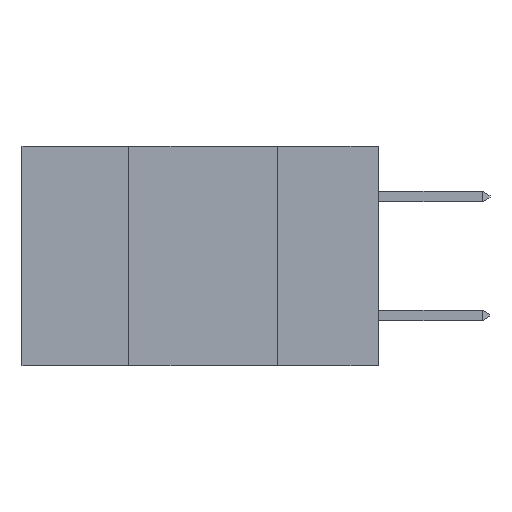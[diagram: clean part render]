
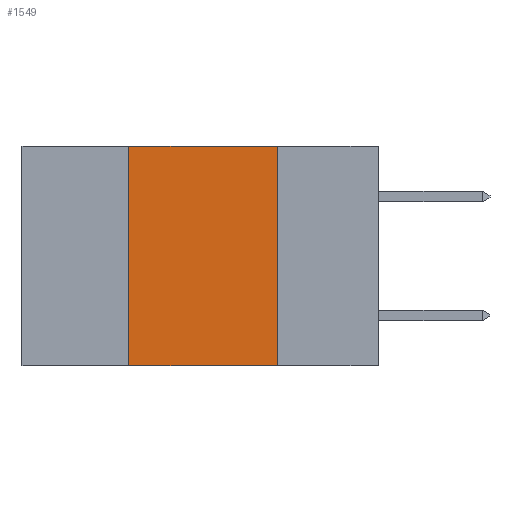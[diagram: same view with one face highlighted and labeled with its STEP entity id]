
A CAD part, left-side view. The second image highlights one B-rep face of the part: STEP entity #1549.
In plain terms, the highlighted planar face has unit normal (-1, 0, 0).
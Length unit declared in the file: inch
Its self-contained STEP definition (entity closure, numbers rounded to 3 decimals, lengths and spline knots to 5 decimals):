
#369 = FACE_OUTER_BOUND ( 'NONE', #4787, .T. ) ;
#428 = EDGE_CURVE ( 'NONE', #509, #7720, #2446, .T. ) ;
#509 = VERTEX_POINT ( 'NONE', #4551 ) ;
#1231 = VECTOR ( 'NONE', #1495, 39.37008 ) ;
#1495 = DIRECTION ( 'NONE',  ( 0., -1., 0. ) ) ;
#1549 = ADVANCED_FACE ( 'NONE', ( #369 ), #8663, .F. ) ;
#1565 = CARTESIAN_POINT ( 'NONE',  ( 0., 0.42, -0.37 ) ) ;
#1822 = LINE ( 'NONE', #11605, #8966 ) ;
#2446 = LINE ( 'NONE', #2611, #5271 ) ;
#2566 = DIRECTION ( 'NONE',  ( 0., 0., -1. ) ) ;
#2611 = CARTESIAN_POINT ( 'NONE',  ( 0., 0.17, 0. ) ) ;
#3352 = CARTESIAN_POINT ( 'NONE',  ( 0., 0.6, 0. ) ) ;
#3728 = CARTESIAN_POINT ( 'NONE',  ( 0., 0.17, -0.37 ) ) ;
#3732 = LINE ( 'NONE', #3352, #1231 ) ;
#4293 = DIRECTION ( 'NONE',  ( 1., 0., 0. ) ) ;
#4511 = VERTEX_POINT ( 'NONE', #6547 ) ;
#4551 = CARTESIAN_POINT ( 'NONE',  ( 0., 0.17, 0. ) ) ;
#4787 = EDGE_LOOP ( 'NONE', ( #9085, #8087, #5956, #11182 ) ) ;
#5271 = VECTOR ( 'NONE', #2566, 39.37008 ) ;
#5327 = EDGE_CURVE ( 'NONE', #8867, #4511, #1822, .T. ) ;
#5956 = ORIENTED_EDGE ( 'NONE', *, *, #5327, .F. ) ;
#6547 = CARTESIAN_POINT ( 'NONE',  ( 0., 0.42, 0. ) ) ;
#6921 = DIRECTION ( 'NONE',  ( 0., 0., 1. ) ) ;
#7214 = CARTESIAN_POINT ( 'NONE',  ( 0., 0.6, 0. ) ) ;
#7720 = VERTEX_POINT ( 'NONE', #3728 ) ;
#7768 = LINE ( 'NONE', #9543, #9960 ) ;
#8087 = ORIENTED_EDGE ( 'NONE', *, *, #9478, .F. ) ;
#8610 = DIRECTION ( 'NONE',  ( 0., -1., 0. ) ) ;
#8663 = PLANE ( 'NONE',  #10232 ) ;
#8867 = VERTEX_POINT ( 'NONE', #1565 ) ;
#8966 = VECTOR ( 'NONE', #6921, 39.37008 ) ;
#9085 = ORIENTED_EDGE ( 'NONE', *, *, #428, .F. ) ;
#9478 = EDGE_CURVE ( 'NONE', #4511, #509, #3732, .T. ) ;
#9543 = CARTESIAN_POINT ( 'NONE',  ( 0., 0.6, -0.37 ) ) ;
#9703 = DIRECTION ( 'NONE',  ( 0., 0., -1. ) ) ;
#9960 = VECTOR ( 'NONE', #8610, 39.37008 ) ;
#10232 = AXIS2_PLACEMENT_3D ( 'NONE', #7214, #4293, #9703 ) ;
#11182 = ORIENTED_EDGE ( 'NONE', *, *, #11541, .T. ) ;
#11541 = EDGE_CURVE ( 'NONE', #8867, #7720, #7768, .T. ) ;
#11605 = CARTESIAN_POINT ( 'NONE',  ( 0., 0.42, 0. ) ) ;
